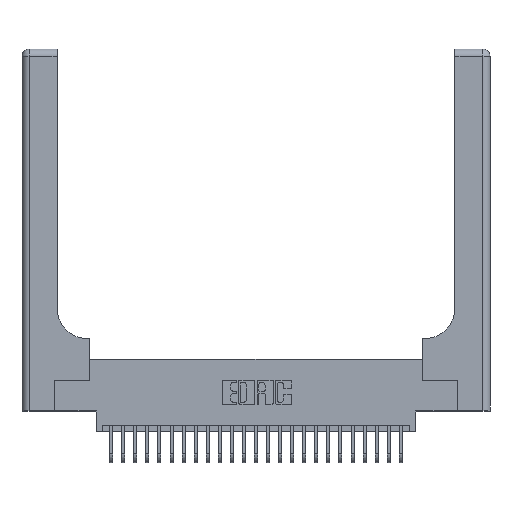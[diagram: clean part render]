
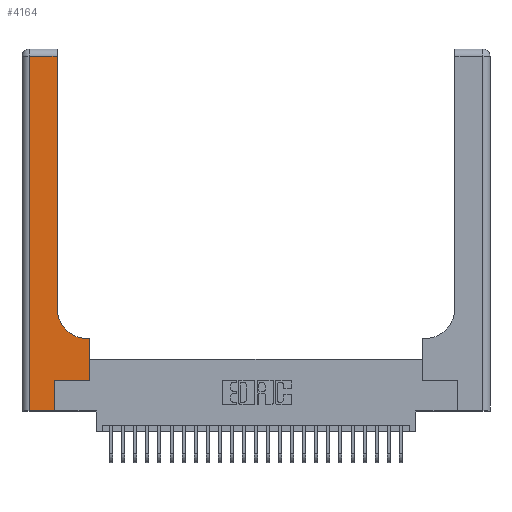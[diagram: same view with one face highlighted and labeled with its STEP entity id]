
A CAD part, top view. The second image highlights one B-rep face of the part: STEP entity #4164.
In plain terms, the highlighted planar face has unit normal (0, 0, 1).
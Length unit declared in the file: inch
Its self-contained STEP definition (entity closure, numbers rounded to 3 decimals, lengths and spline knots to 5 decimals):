
#14 = AXIS2_PLACEMENT_3D ( 'NONE', #2656, #16994, #4729 ) ;
#50 = CARTESIAN_POINT ( 'NONE',  ( 0.5585, 0.25, 0.37 ) ) ;
#231 = ORIENTED_EDGE ( 'NONE', *, *, #17837, .T. ) ;
#1079 = FACE_OUTER_BOUND ( 'NONE', #12354, .T. ) ;
#1795 = LINE ( 'NONE', #16259, #12109 ) ;
#2522 = VECTOR ( 'NONE', #5157, 39.37008 ) ;
#2656 = CARTESIAN_POINT ( 'NONE',  ( 0.5415, 0.85, 0.37 ) ) ;
#2772 = LINE ( 'NONE', #17240, #23843 ) ;
#2885 = ORIENTED_EDGE ( 'NONE', *, *, #10796, .T. ) ;
#2902 = DIRECTION ( 'NONE',  ( -1., 0., 0. ) ) ;
#3340 = ORIENTED_EDGE ( 'NONE', *, *, #19486, .T. ) ;
#3508 = ORIENTED_EDGE ( 'NONE', *, *, #18086, .T. ) ;
#3639 = CARTESIAN_POINT ( 'NONE',  ( 0.269, 0., 0.37 ) ) ;
#4164 = ADVANCED_FACE ( 'NONE', ( #1079 ), #19433, .F. ) ;
#4207 = CARTESIAN_POINT ( 'NONE',  ( 0.269, 0.25, 0.37 ) ) ;
#4729 = DIRECTION ( 'NONE',  ( 1., 0., 0. ) ) ;
#5156 = CARTESIAN_POINT ( 'NONE',  ( 0., 3., 0.37 ) ) ;
#5157 = DIRECTION ( 'NONE',  ( 0., -1., 0. ) ) ;
#5279 = LINE ( 'NONE', #13476, #20916 ) ;
#5654 = ORIENTED_EDGE ( 'NONE', *, *, #18277, .T. ) ;
#5848 = EDGE_CURVE ( 'NONE', #10324, #19834, #21167, .T. ) ;
#6328 = CARTESIAN_POINT ( 'NONE',  ( 0., 0., 0.37 ) ) ;
#6450 = CARTESIAN_POINT ( 'NONE',  ( 0.269, 0., 0.37 ) ) ;
#7642 = CIRCLE ( 'NONE', #14, 0.25 ) ;
#8690 = CARTESIAN_POINT ( 'NONE',  ( 0.2915, 0.85, 0.37 ) ) ;
#9314 = DIRECTION ( 'NONE',  ( -1., 0., 0. ) ) ;
#9807 = CARTESIAN_POINT ( 'NONE',  ( 0.5585, 0.25, 0.37 ) ) ;
#9913 = VERTEX_POINT ( 'NONE', #12468 ) ;
#10324 = VERTEX_POINT ( 'NONE', #3639 ) ;
#10541 = EDGE_CURVE ( 'NONE', #9913, #10324, #16980, .T. ) ;
#10796 = EDGE_CURVE ( 'NONE', #12790, #9913, #13457, .T. ) ;
#11567 = VECTOR ( 'NONE', #18560, 39.37008 ) ;
#11605 = VECTOR ( 'NONE', #22072, 39.37008 ) ;
#11616 = ORIENTED_EDGE ( 'NONE', *, *, #5848, .T. ) ;
#12109 = VECTOR ( 'NONE', #14304, 39.37008 ) ;
#12337 = EDGE_CURVE ( 'NONE', #14093, #18392, #20709, .T. ) ;
#12354 = EDGE_LOOP ( 'NONE', ( #3508, #18381, #2885, #21566, #11616, #3340, #14933, #5654, #231 ) ) ;
#12399 = DIRECTION ( 'NONE',  ( 0., 1., 0. ) ) ;
#12468 = CARTESIAN_POINT ( 'NONE',  ( 0.06, 0., 0.37 ) ) ;
#12715 = DIRECTION ( 'NONE',  ( 0., 1., 0. ) ) ;
#12790 = VERTEX_POINT ( 'NONE', #24003 ) ;
#13351 = LINE ( 'NONE', #20017, #11605 ) ;
#13457 = LINE ( 'NONE', #17421, #2522 ) ;
#13476 = CARTESIAN_POINT ( 'NONE',  ( 0.269, 0.25, 0.37 ) ) ;
#14093 = VERTEX_POINT ( 'NONE', #9807 ) ;
#14304 = DIRECTION ( 'NONE',  ( 0., 1., 0. ) ) ;
#14933 = ORIENTED_EDGE ( 'NONE', *, *, #12337, .T. ) ;
#15345 = VECTOR ( 'NONE', #12399, 39.37008 ) ;
#15399 = VERTEX_POINT ( 'NONE', #24473 ) ;
#15622 = CARTESIAN_POINT ( 'NONE',  ( 0.5585, 0.6, 0.37 ) ) ;
#16259 = CARTESIAN_POINT ( 'NONE',  ( 0.2915, 3., 0.37 ) ) ;
#16980 = LINE ( 'NONE', #6328, #11567 ) ;
#16994 = DIRECTION ( 'NONE',  ( 0., 0., -1. ) ) ;
#17240 = CARTESIAN_POINT ( 'NONE',  ( 0.2915, 0.6, 0.37 ) ) ;
#17421 = CARTESIAN_POINT ( 'NONE',  ( 0.06, 3., 0.37 ) ) ;
#17837 = EDGE_CURVE ( 'NONE', #19074, #23082, #7642, .T. ) ;
#18086 = EDGE_CURVE ( 'NONE', #23082, #15399, #1795, .T. ) ;
#18277 = EDGE_CURVE ( 'NONE', #18392, #19074, #2772, .T. ) ;
#18381 = ORIENTED_EDGE ( 'NONE', *, *, #21511, .T. ) ;
#18392 = VERTEX_POINT ( 'NONE', #15622 ) ;
#18560 = DIRECTION ( 'NONE',  ( 1., 0., 0. ) ) ;
#19074 = VERTEX_POINT ( 'NONE', #26104 ) ;
#19433 = PLANE ( 'NONE',  #26288 ) ;
#19486 = EDGE_CURVE ( 'NONE', #19834, #14093, #5279, .T. ) ;
#19834 = VERTEX_POINT ( 'NONE', #4207 ) ;
#20017 = CARTESIAN_POINT ( 'NONE',  ( 0., 2.94, 0.37 ) ) ;
#20518 = VECTOR ( 'NONE', #12715, 39.37008 ) ;
#20709 = LINE ( 'NONE', #50, #15345 ) ;
#20916 = VECTOR ( 'NONE', #25628, 39.37008 ) ;
#21167 = LINE ( 'NONE', #6450, #20518 ) ;
#21476 = DIRECTION ( 'NONE',  ( 0., 0., -1. ) ) ;
#21511 = EDGE_CURVE ( 'NONE', #15399, #12790, #13351, .T. ) ;
#21566 = ORIENTED_EDGE ( 'NONE', *, *, #10541, .T. ) ;
#22072 = DIRECTION ( 'NONE',  ( -1., 0., 0. ) ) ;
#23082 = VERTEX_POINT ( 'NONE', #8690 ) ;
#23843 = VECTOR ( 'NONE', #2902, 39.37008 ) ;
#24003 = CARTESIAN_POINT ( 'NONE',  ( 0.06, 2.94, 0.37 ) ) ;
#24473 = CARTESIAN_POINT ( 'NONE',  ( 0.2915, 2.94, 0.37 ) ) ;
#25628 = DIRECTION ( 'NONE',  ( 1., 0., 0. ) ) ;
#26104 = CARTESIAN_POINT ( 'NONE',  ( 0.5415, 0.6, 0.37 ) ) ;
#26288 = AXIS2_PLACEMENT_3D ( 'NONE', #5156, #21476, #9314 ) ;
